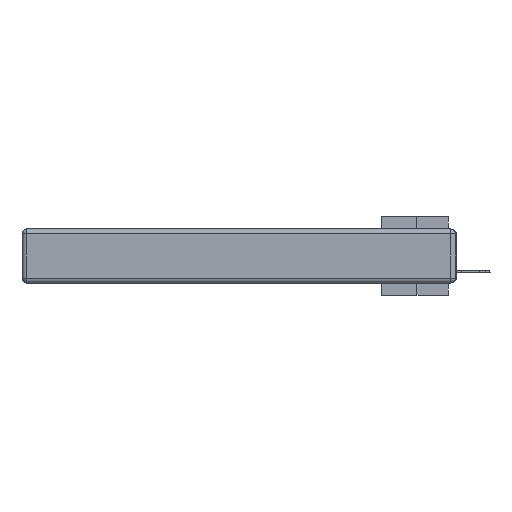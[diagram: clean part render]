
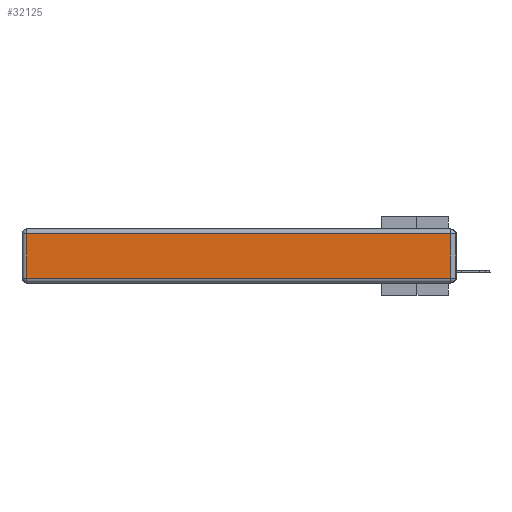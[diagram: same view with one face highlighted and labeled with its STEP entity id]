
A CAD part, left-side view. The second image highlights one B-rep face of the part: STEP entity #32125.
In plain terms, the highlighted planar face has unit normal (-1, 0, 0).
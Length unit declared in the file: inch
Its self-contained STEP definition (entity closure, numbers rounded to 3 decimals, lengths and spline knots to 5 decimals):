
#206 = VECTOR ( 'NONE', #26154, 39.37008 ) ;
#659 = VECTOR ( 'NONE', #27017, 39.37008 ) ;
#926 = VERTEX_POINT ( 'NONE', #10931 ) ;
#3591 = ORIENTED_EDGE ( 'NONE', *, *, #21005, .T. ) ;
#5934 = CARTESIAN_POINT ( 'NONE',  ( 0., 2.72, -0.313 ) ) ;
#6956 = EDGE_CURVE ( 'NONE', #26414, #9545, #9249, .T. ) ;
#6969 = DIRECTION ( 'NONE',  ( -1., 0., 0. ) ) ;
#7506 = AXIS2_PLACEMENT_3D ( 'NONE', #29292, #6969, #23932 ) ;
#9226 = LINE ( 'NONE', #28965, #16230 ) ;
#9249 = LINE ( 'NONE', #27175, #659 ) ;
#9422 = EDGE_CURVE ( 'NONE', #18595, #26414, #18813, .T. ) ;
#9545 = VERTEX_POINT ( 'NONE', #19135 ) ;
#10931 = CARTESIAN_POINT ( 'NONE',  ( 0., 2.72, -0.03 ) ) ;
#11153 = DIRECTION ( 'NONE',  ( 0., -1., 0. ) ) ;
#12569 = ORIENTED_EDGE ( 'NONE', *, *, #18309, .T. ) ;
#13759 = CARTESIAN_POINT ( 'NONE',  ( 0., 0., -0.313 ) ) ;
#16224 = LINE ( 'NONE', #26006, #206 ) ;
#16230 = VECTOR ( 'NONE', #31566, 39.37008 ) ;
#18309 = EDGE_CURVE ( 'NONE', #926, #18595, #9226, .T. ) ;
#18595 = VERTEX_POINT ( 'NONE', #5934 ) ;
#18813 = LINE ( 'NONE', #13759, #24776 ) ;
#19135 = CARTESIAN_POINT ( 'NONE',  ( 0., 0.03, -0.03 ) ) ;
#20843 = EDGE_LOOP ( 'NONE', ( #30661, #26308, #3591, #12569 ) ) ;
#21005 = EDGE_CURVE ( 'NONE', #9545, #926, #16224, .T. ) ;
#23681 = CARTESIAN_POINT ( 'NONE',  ( 0., 0.03, -0.313 ) ) ;
#23932 = DIRECTION ( 'NONE',  ( 0., 0., 1. ) ) ;
#24776 = VECTOR ( 'NONE', #11153, 39.37008 ) ;
#26006 = CARTESIAN_POINT ( 'NONE',  ( 0., 2.75, -0.03 ) ) ;
#26154 = DIRECTION ( 'NONE',  ( 0., 1., 0. ) ) ;
#26308 = ORIENTED_EDGE ( 'NONE', *, *, #6956, .T. ) ;
#26414 = VERTEX_POINT ( 'NONE', #23681 ) ;
#27017 = DIRECTION ( 'NONE',  ( 0., 0., 1. ) ) ;
#27175 = CARTESIAN_POINT ( 'NONE',  ( 0., 0.03, -0.343 ) ) ;
#28965 = CARTESIAN_POINT ( 'NONE',  ( 0., 2.72, -0.343 ) ) ;
#29292 = CARTESIAN_POINT ( 'NONE',  ( 0., 0., -0.343 ) ) ;
#30661 = ORIENTED_EDGE ( 'NONE', *, *, #9422, .T. ) ;
#31265 = PLANE ( 'NONE',  #7506 ) ;
#31566 = DIRECTION ( 'NONE',  ( 0., 0., -1. ) ) ;
#31744 = FACE_OUTER_BOUND ( 'NONE', #20843, .T. ) ;
#32125 = ADVANCED_FACE ( 'NONE', ( #31744 ), #31265, .T. ) ;
